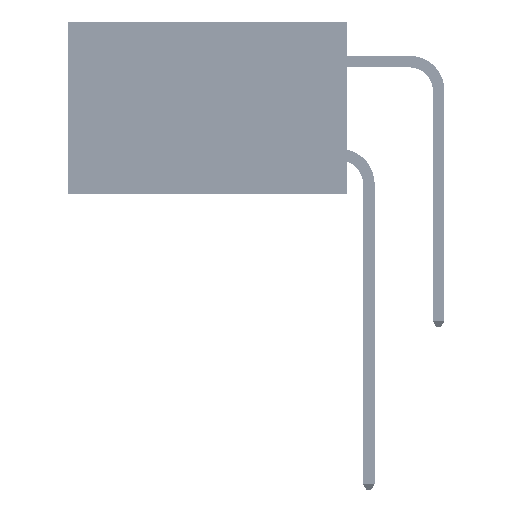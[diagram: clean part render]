
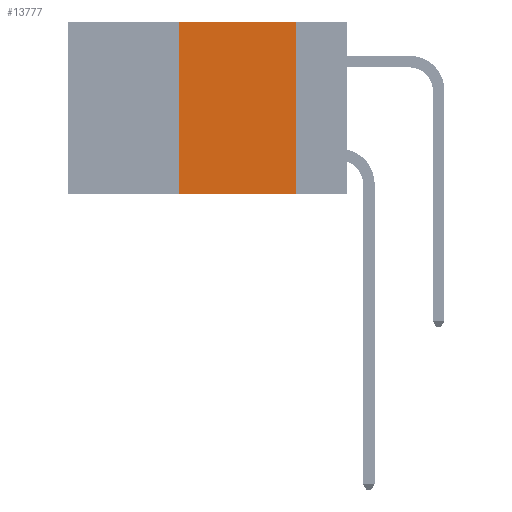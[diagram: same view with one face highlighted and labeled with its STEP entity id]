
A CAD part, left-side view. The second image highlights one B-rep face of the part: STEP entity #13777.
In plain terms, the highlighted planar face has unit normal (-1, 0, 0).
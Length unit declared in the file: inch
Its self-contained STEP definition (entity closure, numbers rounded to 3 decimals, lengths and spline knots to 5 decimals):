
#2054 = VECTOR ( 'NONE', #39467, 39.37008 ) ;
#3371 = ORIENTED_EDGE ( 'NONE', *, *, #6866, .F. ) ;
#6866 = EDGE_CURVE ( 'NONE', #16075, #35177, #29722, .T. ) ;
#7921 = ORIENTED_EDGE ( 'NONE', *, *, #36298, .F. ) ;
#8151 = DIRECTION ( 'NONE',  ( 0., 0., 1. ) ) ;
#8261 = FACE_OUTER_BOUND ( 'NONE', #38374, .T. ) ;
#8407 = CARTESIAN_POINT ( 'NONE',  ( 0., 0.6, -0.37 ) ) ;
#9076 = PLANE ( 'NONE',  #50695 ) ;
#9240 = DIRECTION ( 'NONE',  ( 0., 0., -1. ) ) ;
#12862 = VERTEX_POINT ( 'NONE', #41910 ) ;
#13777 = ADVANCED_FACE ( 'NONE', ( #8261 ), #9076, .F. ) ;
#14660 = CARTESIAN_POINT ( 'NONE',  ( 0., 0.36, 0. ) ) ;
#15583 = EDGE_CURVE ( 'NONE', #12862, #16075, #37593, .T. ) ;
#16075 = VERTEX_POINT ( 'NONE', #14660 ) ;
#16794 = DIRECTION ( 'NONE',  ( 1., 0., 0. ) ) ;
#17464 = DIRECTION ( 'NONE',  ( 0., 0., -1. ) ) ;
#23525 = ORIENTED_EDGE ( 'NONE', *, *, #15583, .F. ) ;
#24073 = CARTESIAN_POINT ( 'NONE',  ( 0., 0.11, 0. ) ) ;
#24649 = VECTOR ( 'NONE', #8151, 39.37008 ) ;
#29034 = EDGE_CURVE ( 'NONE', #12862, #42347, #36240, .T. ) ;
#29722 = LINE ( 'NONE', #43589, #2054 ) ;
#31951 = DIRECTION ( 'NONE',  ( 0., -1., 0. ) ) ;
#33423 = CARTESIAN_POINT ( 'NONE',  ( 0., 0.11, -0.37 ) ) ;
#33769 = VECTOR ( 'NONE', #31951, 39.37008 ) ;
#35177 = VERTEX_POINT ( 'NONE', #24073 ) ;
#36082 = ORIENTED_EDGE ( 'NONE', *, *, #29034, .T. ) ;
#36240 = LINE ( 'NONE', #8407, #33769 ) ;
#36298 = EDGE_CURVE ( 'NONE', #35177, #42347, #36714, .T. ) ;
#36714 = LINE ( 'NONE', #41567, #45341 ) ;
#37593 = LINE ( 'NONE', #39967, #24649 ) ;
#38374 = EDGE_LOOP ( 'NONE', ( #7921, #3371, #23525, #36082 ) ) ;
#39467 = DIRECTION ( 'NONE',  ( 0., -1., 0. ) ) ;
#39967 = CARTESIAN_POINT ( 'NONE',  ( 0., 0.36, 0. ) ) ;
#41567 = CARTESIAN_POINT ( 'NONE',  ( 0., 0.11, 0. ) ) ;
#41910 = CARTESIAN_POINT ( 'NONE',  ( 0., 0.36, -0.37 ) ) ;
#42347 = VERTEX_POINT ( 'NONE', #33423 ) ;
#43589 = CARTESIAN_POINT ( 'NONE',  ( 0., 0.6, 0. ) ) ;
#44670 = CARTESIAN_POINT ( 'NONE',  ( 0., 0.6, 0. ) ) ;
#45341 = VECTOR ( 'NONE', #17464, 39.37008 ) ;
#50695 = AXIS2_PLACEMENT_3D ( 'NONE', #44670, #16794, #9240 ) ;
